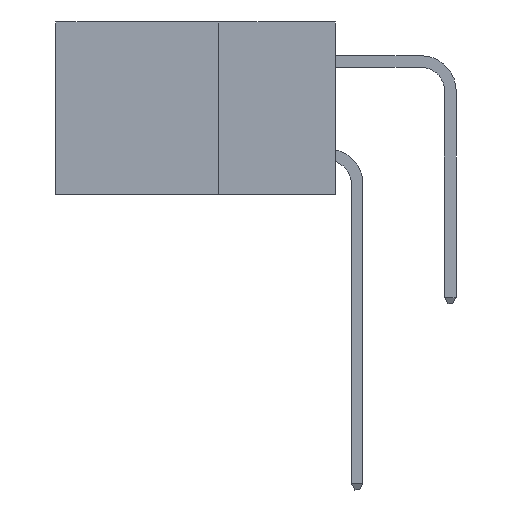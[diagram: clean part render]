
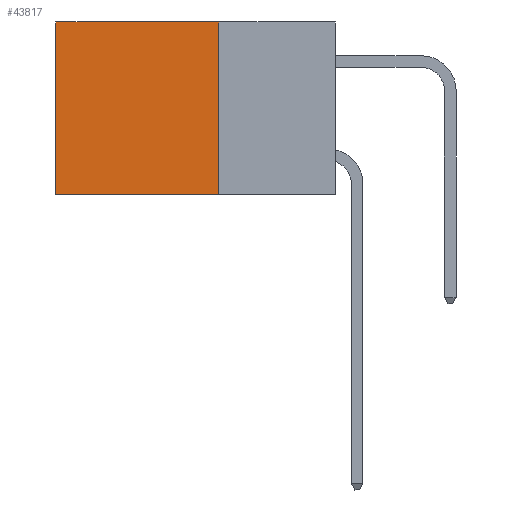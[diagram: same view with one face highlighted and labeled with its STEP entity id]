
A CAD part, left-side view. The second image highlights one B-rep face of the part: STEP entity #43817.
In plain terms, the highlighted planar face has unit normal (-1, 0, 0).
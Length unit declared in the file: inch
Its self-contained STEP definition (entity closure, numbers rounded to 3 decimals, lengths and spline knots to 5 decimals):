
#1519 = VECTOR ( 'NONE', #36821, 39.37008 ) ;
#4146 = EDGE_CURVE ( 'NONE', #17684, #38127, #4451, .T. ) ;
#4451 = LINE ( 'NONE', #7721, #25937 ) ;
#5519 = DIRECTION ( 'NONE',  ( 0., 0., -1. ) ) ;
#6092 = ORIENTED_EDGE ( 'NONE', *, *, #42353, .T. ) ;
#6197 = LINE ( 'NONE', #41572, #36158 ) ;
#6460 = PLANE ( 'NONE',  #9220 ) ;
#7721 = CARTESIAN_POINT ( 'NONE',  ( 0.2875, 0.25, 0. ) ) ;
#8384 = LINE ( 'NONE', #43006, #29783 ) ;
#9220 = AXIS2_PLACEMENT_3D ( 'NONE', #30520, #40797, #43933 ) ;
#11570 = DIRECTION ( 'NONE',  ( 0., 1., 0. ) ) ;
#12372 = EDGE_LOOP ( 'NONE', ( #6092, #12415, #23290, #26027 ) ) ;
#12415 = ORIENTED_EDGE ( 'NONE', *, *, #36451, .F. ) ;
#12633 = VERTEX_POINT ( 'NONE', #16342 ) ;
#14391 = VERTEX_POINT ( 'NONE', #21159 ) ;
#16342 = CARTESIAN_POINT ( 'NONE',  ( 0.2875, 0.6, -0.37 ) ) ;
#17684 = VERTEX_POINT ( 'NONE', #18201 ) ;
#18201 = CARTESIAN_POINT ( 'NONE',  ( 0.2875, 0.25, 0. ) ) ;
#18379 = FACE_OUTER_BOUND ( 'NONE', #12372, .T. ) ;
#19950 = CARTESIAN_POINT ( 'NONE',  ( 0.2875, 0.25, -0.37 ) ) ;
#21159 = CARTESIAN_POINT ( 'NONE',  ( 0.2875, 0.6, 0. ) ) ;
#22977 = LINE ( 'NONE', #40102, #1519 ) ;
#23290 = ORIENTED_EDGE ( 'NONE', *, *, #4146, .F. ) ;
#25937 = VECTOR ( 'NONE', #35360, 39.37008 ) ;
#26027 = ORIENTED_EDGE ( 'NONE', *, *, #34835, .T. ) ;
#29783 = VECTOR ( 'NONE', #5519, 39.37008 ) ;
#30520 = CARTESIAN_POINT ( 'NONE',  ( 0.2875, 0.25, 0. ) ) ;
#34835 = EDGE_CURVE ( 'NONE', #17684, #14391, #22977, .T. ) ;
#35360 = DIRECTION ( 'NONE',  ( 0., 0., -1. ) ) ;
#36158 = VECTOR ( 'NONE', #11570, 39.37008 ) ;
#36451 = EDGE_CURVE ( 'NONE', #38127, #12633, #6197, .T. ) ;
#36821 = DIRECTION ( 'NONE',  ( 0., 1., 0. ) ) ;
#38127 = VERTEX_POINT ( 'NONE', #19950 ) ;
#40102 = CARTESIAN_POINT ( 'NONE',  ( 0.2875, 0.25, 0. ) ) ;
#40797 = DIRECTION ( 'NONE',  ( 1., 0., 0. ) ) ;
#41572 = CARTESIAN_POINT ( 'NONE',  ( 0.2875, 0.25, -0.37 ) ) ;
#42353 = EDGE_CURVE ( 'NONE', #14391, #12633, #8384, .T. ) ;
#43006 = CARTESIAN_POINT ( 'NONE',  ( 0.2875, 0.6, 0. ) ) ;
#43817 = ADVANCED_FACE ( 'NONE', ( #18379 ), #6460, .F. ) ;
#43933 = DIRECTION ( 'NONE',  ( 0., 0., -1. ) ) ;
